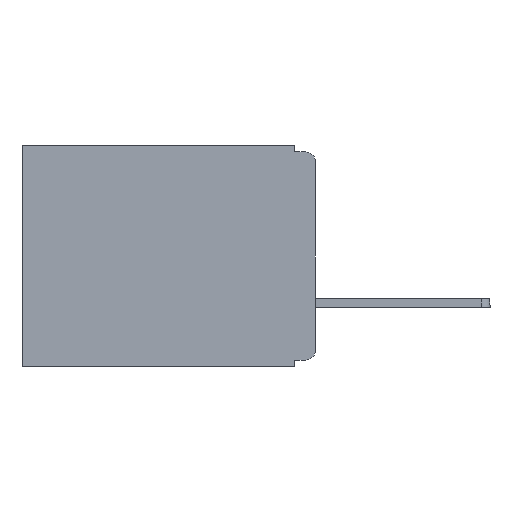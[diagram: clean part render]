
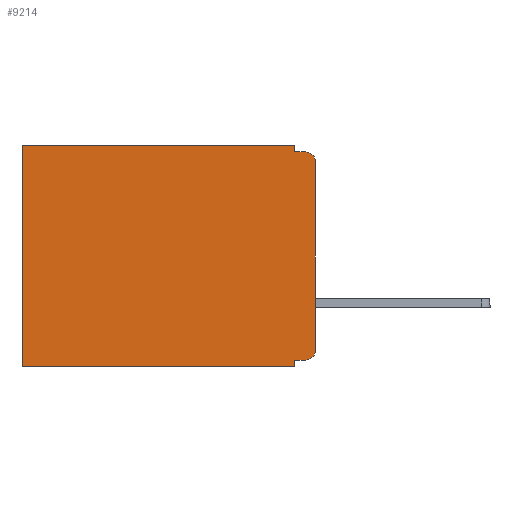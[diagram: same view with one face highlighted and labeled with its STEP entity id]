
A CAD part, left-side view. The second image highlights one B-rep face of the part: STEP entity #9214.
In plain terms, the highlighted planar face has unit normal (-1, 0, 0).
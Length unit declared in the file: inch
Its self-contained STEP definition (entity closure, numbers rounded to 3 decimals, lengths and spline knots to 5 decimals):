
#44 = EDGE_CURVE ( 'NONE', #20927, #28039, #9818, .T. ) ;
#166 = CARTESIAN_POINT ( 'NONE',  ( 0.3, 0., -0.025 ) ) ;
#265 = AXIS2_PLACEMENT_3D ( 'NONE', #28636, #15261, #1570 ) ;
#469 = ORIENTED_EDGE ( 'NONE', *, *, #17435, .T. ) ;
#603 = LINE ( 'NONE', #8471, #6006 ) ;
#1230 = ORIENTED_EDGE ( 'NONE', *, *, #4991, .F. ) ;
#1570 = DIRECTION ( 'NONE',  ( 0., 0., -1. ) ) ;
#1822 = AXIS2_PLACEMENT_3D ( 'NONE', #17140, #3510, #19370 ) ;
#2434 = FACE_OUTER_BOUND ( 'NONE', #17457, .T. ) ;
#2797 = CARTESIAN_POINT ( 'NONE',  ( 0.3, 0., 0. ) ) ;
#2936 = VECTOR ( 'NONE', #7101, 39.37008 ) ;
#2938 = CARTESIAN_POINT ( 'NONE',  ( 0.3, 0.031, -0.01 ) ) ;
#2943 = CARTESIAN_POINT ( 'NONE',  ( 0.3, 0.437, -0.33 ) ) ;
#3035 = ORIENTED_EDGE ( 'NONE', *, *, #19606, .F. ) ;
#3492 = DIRECTION ( 'NONE',  ( 0., -1., 0. ) ) ;
#3510 = DIRECTION ( 'NONE',  ( -1., 0., 0. ) ) ;
#3544 = DIRECTION ( 'NONE',  ( 0., 0., -1. ) ) ;
#3664 = VECTOR ( 'NONE', #5755, 39.37008 ) ;
#3929 = EDGE_CURVE ( 'NONE', #28039, #18508, #19748, .T. ) ;
#4098 = ORIENTED_EDGE ( 'NONE', *, *, #20202, .F. ) ;
#4352 = CARTESIAN_POINT ( 'NONE',  ( 0.3, 0., -0.33 ) ) ;
#4991 = EDGE_CURVE ( 'NONE', #21777, #14620, #16219, .T. ) ;
#5755 = DIRECTION ( 'NONE',  ( 0., 1., 0. ) ) ;
#6006 = VECTOR ( 'NONE', #26434, 39.37008 ) ;
#6355 = CARTESIAN_POINT ( 'NONE',  ( 0.3, 0.015, -0.32 ) ) ;
#6571 = AXIS2_PLACEMENT_3D ( 'NONE', #4352, #9024, #24754 ) ;
#7101 = DIRECTION ( 'NONE',  ( 0., 0., -1. ) ) ;
#7246 = EDGE_CURVE ( 'NONE', #14620, #17778, #20311, .T. ) ;
#7584 = CARTESIAN_POINT ( 'NONE',  ( 0.3, 0.031, -0.33 ) ) ;
#8069 = CARTESIAN_POINT ( 'NONE',  ( 0.3, 0., -0.01 ) ) ;
#8104 = VERTEX_POINT ( 'NONE', #166 ) ;
#8471 = CARTESIAN_POINT ( 'NONE',  ( 0.3, 0., -0.33 ) ) ;
#9024 = DIRECTION ( 'NONE',  ( 1., 0., 0. ) ) ;
#9154 = VERTEX_POINT ( 'NONE', #28895 ) ;
#9214 = ADVANCED_FACE ( 'NONE', ( #2434 ), #22485, .F. ) ;
#9446 = VERTEX_POINT ( 'NONE', #2938 ) ;
#9818 = LINE ( 'NONE', #2797, #3664 ) ;
#10013 = CIRCLE ( 'NONE', #265, 0.015 ) ;
#10464 = DIRECTION ( 'NONE',  ( 0., 1., 0. ) ) ;
#12501 = CARTESIAN_POINT ( 'NONE',  ( 0.3, 0.015, -0.01 ) ) ;
#12712 = CARTESIAN_POINT ( 'NONE',  ( 0.3, 0., -0.33 ) ) ;
#12843 = CIRCLE ( 'NONE', #1822, 0.015 ) ;
#13806 = CARTESIAN_POINT ( 'NONE',  ( 0.3, 0.031, -0.33 ) ) ;
#13816 = VECTOR ( 'NONE', #20132, 39.37008 ) ;
#14151 = ORIENTED_EDGE ( 'NONE', *, *, #26692, .T. ) ;
#14405 = LINE ( 'NONE', #17169, #26319 ) ;
#14620 = VERTEX_POINT ( 'NONE', #21659 ) ;
#14806 = ORIENTED_EDGE ( 'NONE', *, *, #22262, .F. ) ;
#15173 = CARTESIAN_POINT ( 'NONE',  ( 0.3, 0.031, 0. ) ) ;
#15261 = DIRECTION ( 'NONE',  ( -1., 0., 0. ) ) ;
#15699 = VERTEX_POINT ( 'NONE', #12501 ) ;
#15881 = ORIENTED_EDGE ( 'NONE', *, *, #7246, .F. ) ;
#16219 = LINE ( 'NONE', #17261, #28097 ) ;
#16267 = CARTESIAN_POINT ( 'NONE',  ( 0.3, 0.437, -0.33 ) ) ;
#17140 = CARTESIAN_POINT ( 'NONE',  ( 0.3, 0.015, -0.025 ) ) ;
#17169 = CARTESIAN_POINT ( 'NONE',  ( 0.3, 0.031, 0. ) ) ;
#17261 = CARTESIAN_POINT ( 'NONE',  ( 0.3, 0., -0.32 ) ) ;
#17435 = EDGE_CURVE ( 'NONE', #8104, #15699, #12843, .T. ) ;
#17457 = EDGE_LOOP ( 'NONE', ( #28826, #469, #14806, #4098, #28789, #19719, #3035, #15881, #1230, #14151 ) ) ;
#17778 = VERTEX_POINT ( 'NONE', #13806 ) ;
#18508 = VERTEX_POINT ( 'NONE', #2943 ) ;
#19370 = DIRECTION ( 'NONE',  ( 0., 0., -1. ) ) ;
#19606 = EDGE_CURVE ( 'NONE', #17778, #18508, #24629, .T. ) ;
#19719 = ORIENTED_EDGE ( 'NONE', *, *, #3929, .T. ) ;
#19748 = LINE ( 'NONE', #16267, #13816 ) ;
#20132 = DIRECTION ( 'NONE',  ( 0., 0., -1. ) ) ;
#20202 = EDGE_CURVE ( 'NONE', #20927, #9446, #14405, .T. ) ;
#20311 = LINE ( 'NONE', #7584, #2936 ) ;
#20456 = VECTOR ( 'NONE', #3492, 39.37008 ) ;
#20927 = VERTEX_POINT ( 'NONE', #15173 ) ;
#21659 = CARTESIAN_POINT ( 'NONE',  ( 0.3, 0.031, -0.32 ) ) ;
#21777 = VERTEX_POINT ( 'NONE', #6355 ) ;
#22262 = EDGE_CURVE ( 'NONE', #9446, #15699, #26425, .T. ) ;
#22485 = PLANE ( 'NONE',  #6571 ) ;
#23925 = VECTOR ( 'NONE', #10464, 39.37008 ) ;
#24629 = LINE ( 'NONE', #12712, #23925 ) ;
#24664 = DIRECTION ( 'NONE',  ( 0., 1., 0. ) ) ;
#24754 = DIRECTION ( 'NONE',  ( 0., 0., -1. ) ) ;
#26319 = VECTOR ( 'NONE', #3544, 39.37008 ) ;
#26425 = LINE ( 'NONE', #8069, #20456 ) ;
#26434 = DIRECTION ( 'NONE',  ( 0., 0., -1. ) ) ;
#26673 = CARTESIAN_POINT ( 'NONE',  ( 0.3, 0.437, 0. ) ) ;
#26692 = EDGE_CURVE ( 'NONE', #21777, #9154, #10013, .T. ) ;
#28039 = VERTEX_POINT ( 'NONE', #26673 ) ;
#28097 = VECTOR ( 'NONE', #24664, 39.37008 ) ;
#28636 = CARTESIAN_POINT ( 'NONE',  ( 0.3, 0.015, -0.305 ) ) ;
#28789 = ORIENTED_EDGE ( 'NONE', *, *, #44, .T. ) ;
#28826 = ORIENTED_EDGE ( 'NONE', *, *, #29079, .F. ) ;
#28895 = CARTESIAN_POINT ( 'NONE',  ( 0.3, 0., -0.305 ) ) ;
#29079 = EDGE_CURVE ( 'NONE', #8104, #9154, #603, .T. ) ;
